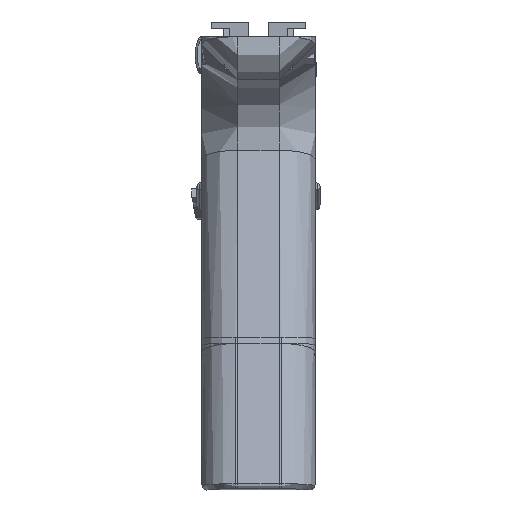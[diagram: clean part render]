
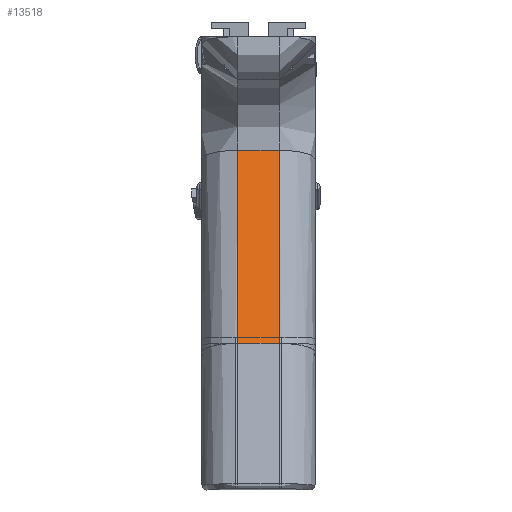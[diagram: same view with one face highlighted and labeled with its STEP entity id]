
A CAD part, front view. The second image highlights one B-rep face of the part: STEP entity #13518.
In plain terms, the highlighted face is planar.
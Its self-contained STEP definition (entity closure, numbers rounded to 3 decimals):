
#974=PLANE('',#14702);
#1571=FACE_OUTER_BOUND('',#2356,.T.);
#2356=EDGE_LOOP('',(#11317,#11318,#11319,#11320));
#3356=LINE('',#22664,#4605);
#3510=LINE('',#23509,#4759);
#3511=LINE('',#23512,#4760);
#3512=LINE('',#23513,#4761);
#4605=VECTOR('',#17133,10.);
#4759=VECTOR('',#17533,10.);
#4760=VECTOR('',#17536,10.);
#4761=VECTOR('',#17537,10.);
#6259=VERTEX_POINT('',#22660);
#6260=VERTEX_POINT('',#22662);
#6395=VERTEX_POINT('',#23487);
#6398=VERTEX_POINT('',#23511);
#7912=EDGE_CURVE('',#6259,#6260,#3356,.T.);
#8136=EDGE_CURVE('',#6259,#6395,#3510,.T.);
#8137=EDGE_CURVE('',#6398,#6260,#3511,.T.);
#8138=EDGE_CURVE('',#6395,#6398,#3512,.T.);
#11317=ORIENTED_EDGE('',*,*,#8137,.F.);
#11318=ORIENTED_EDGE('',*,*,#8138,.F.);
#11319=ORIENTED_EDGE('',*,*,#8136,.F.);
#11320=ORIENTED_EDGE('',*,*,#7912,.T.);
#13518=ADVANCED_FACE('',(#1571),#974,.T.);
#14702=AXIS2_PLACEMENT_3D('',#23510,#17534,#17535);
#17133=DIRECTION('',(0.,-0.249,0.969));
#17533=DIRECTION('',(-1.,0.,0.));
#17534=DIRECTION('center_axis',(0.,-0.969,
-0.249));
#17535=DIRECTION('ref_axis',(0.,-0.249,0.969));
#17536=DIRECTION('',(1.,0.,0.));
#17537=DIRECTION('',(0.,-0.249,0.969));
#22660=CARTESIAN_POINT('',(13.45,-71.634,19.877));
#22662=CARTESIAN_POINT('',(13.45,-83.628,66.536));
#22664=CARTESIAN_POINT('',(13.45,-83.554,66.245));
#23487=CARTESIAN_POINT('',(3.45,-71.634,19.877));
#23509=CARTESIAN_POINT('',(22.175,-71.634,19.877));
#23510=CARTESIAN_POINT('Origin',(22.175,-71.634,19.877));
#23511=CARTESIAN_POINT('',(3.45,-83.628,66.536));
#23512=CARTESIAN_POINT('',(22.175,-83.628,66.536));
#23513=CARTESIAN_POINT('',(3.45,-83.554,66.245));
